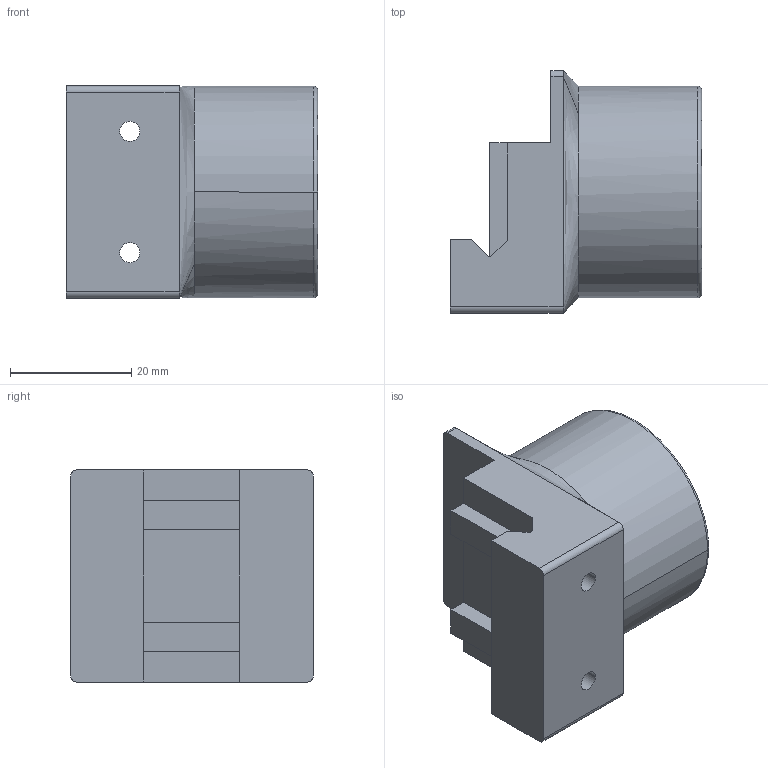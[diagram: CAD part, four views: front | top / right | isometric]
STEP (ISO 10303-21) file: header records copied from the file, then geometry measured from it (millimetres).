
FILE_DESCRIPTION (( 'STEP AP203' ), '1' );
FILE_NAME ('3_4 BSPT Rail Adapter.STEP', '2020-10-26T18:05:00', ( '' ), ( '' ), 'SwSTEP 2.0', 'SolidWorks 2019', '' );
FILE_SCHEMA (( 'CONFIG_CONTROL_DESIGN' ));
Length unit declared in the file: inch
Products named in the file (1): 3_4 BSPT Rail Adapter
Bounding box: 41.46 x 40 x 35 mm (x, y, z)
Volume: 27728.3 mm3; surface area: 9827.1 mm2
Topology: 1 solids, 1 shells, 63 faces, 172 edges, 112 vertices
Faces by surface type: plane 23, cone 20, cylinder 13, bspline 5, torus 2
Entity records: 5482 total; most frequent: CARTESIAN_POINT 3857, ORIENTED_EDGE 344, DIRECTION 291, EDGE_CURVE 172, VERTEX_POINT 112, AXIS2_PLACEMENT_3D 102, VECTOR 87, LINE 87
